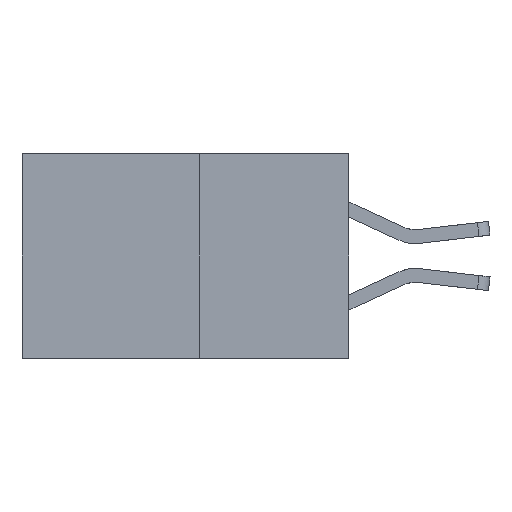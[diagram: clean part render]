
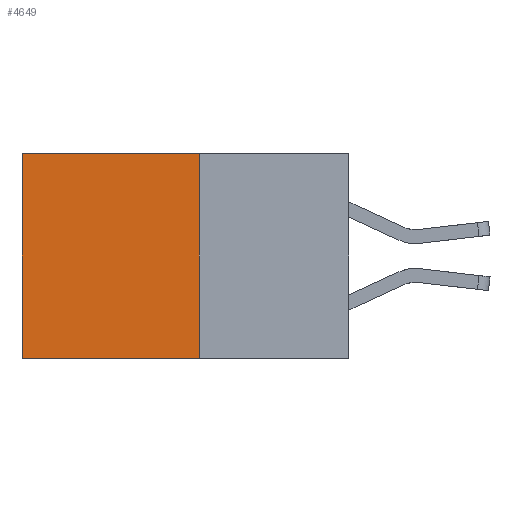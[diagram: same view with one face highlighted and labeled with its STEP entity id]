
A CAD part, left-side view. The second image highlights one B-rep face of the part: STEP entity #4649.
In plain terms, the highlighted planar face has unit normal (-1, 0, 0).
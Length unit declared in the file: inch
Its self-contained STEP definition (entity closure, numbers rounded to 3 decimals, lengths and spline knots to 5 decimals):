
#532 = DIRECTION ( 'NONE',  ( 0., 1., 0. ) ) ;
#1043 = CARTESIAN_POINT ( 'NONE',  ( 0.277, 0.59, 0. ) ) ;
#1064 = LINE ( 'NONE', #3638, #2387 ) ;
#1083 = CARTESIAN_POINT ( 'NONE',  ( 0.277, 0.27, -0.37 ) ) ;
#1148 = PLANE ( 'NONE',  #4676 ) ;
#1272 = CARTESIAN_POINT ( 'NONE',  ( 0.277, 0.27, 0. ) ) ;
#1557 = EDGE_CURVE ( 'NONE', #3577, #3167, #1064, .T. ) ;
#1848 = DIRECTION ( 'NONE',  ( 0., 0., -1. ) ) ;
#1857 = DIRECTION ( 'NONE',  ( 1., 0., 0. ) ) ;
#2387 = VECTOR ( 'NONE', #532, 39.37008 ) ;
#2428 = CARTESIAN_POINT ( 'NONE',  ( 0.277, 0.27, 0. ) ) ;
#2755 = FACE_OUTER_BOUND ( 'NONE', #4528, .T. ) ;
#2996 = ORIENTED_EDGE ( 'NONE', *, *, #4150, .T. ) ;
#3073 = ORIENTED_EDGE ( 'NONE', *, *, #1557, .F. ) ;
#3167 = VERTEX_POINT ( 'NONE', #3588 ) ;
#3233 = LINE ( 'NONE', #7542, #4330 ) ;
#3278 = ORIENTED_EDGE ( 'NONE', *, *, #5171, .F. ) ;
#3431 = VECTOR ( 'NONE', #7573, 39.37008 ) ;
#3457 = ORIENTED_EDGE ( 'NONE', *, *, #3509, .T. ) ;
#3509 = EDGE_CURVE ( 'NONE', #7521, #7427, #4438, .T. ) ;
#3577 = VERTEX_POINT ( 'NONE', #5430 ) ;
#3588 = CARTESIAN_POINT ( 'NONE',  ( 0.277, 0.59, -0.37 ) ) ;
#3638 = CARTESIAN_POINT ( 'NONE',  ( 0.277, 0.27, -0.37 ) ) ;
#4150 = EDGE_CURVE ( 'NONE', #7427, #3167, #3233, .T. ) ;
#4330 = VECTOR ( 'NONE', #7699, 39.37008 ) ;
#4438 = LINE ( 'NONE', #1272, #5897 ) ;
#4528 = EDGE_LOOP ( 'NONE', ( #2996, #3073, #3278, #3457 ) ) ;
#4649 = ADVANCED_FACE ( 'NONE', ( #2755 ), #1148, .F. ) ;
#4676 = AXIS2_PLACEMENT_3D ( 'NONE', #1083, #1857, #1848 ) ;
#5150 = DIRECTION ( 'NONE',  ( 0., 1., 0. ) ) ;
#5171 = EDGE_CURVE ( 'NONE', #7521, #3577, #5679, .T. ) ;
#5430 = CARTESIAN_POINT ( 'NONE',  ( 0.277, 0.27, -0.37 ) ) ;
#5679 = LINE ( 'NONE', #7545, #3431 ) ;
#5897 = VECTOR ( 'NONE', #5150, 39.37008 ) ;
#7427 = VERTEX_POINT ( 'NONE', #1043 ) ;
#7521 = VERTEX_POINT ( 'NONE', #2428 ) ;
#7542 = CARTESIAN_POINT ( 'NONE',  ( 0.277, 0.59, -0.37 ) ) ;
#7545 = CARTESIAN_POINT ( 'NONE',  ( 0.277, 0.27, -0.37 ) ) ;
#7573 = DIRECTION ( 'NONE',  ( 0., 0., -1. ) ) ;
#7699 = DIRECTION ( 'NONE',  ( 0., 0., -1. ) ) ;
